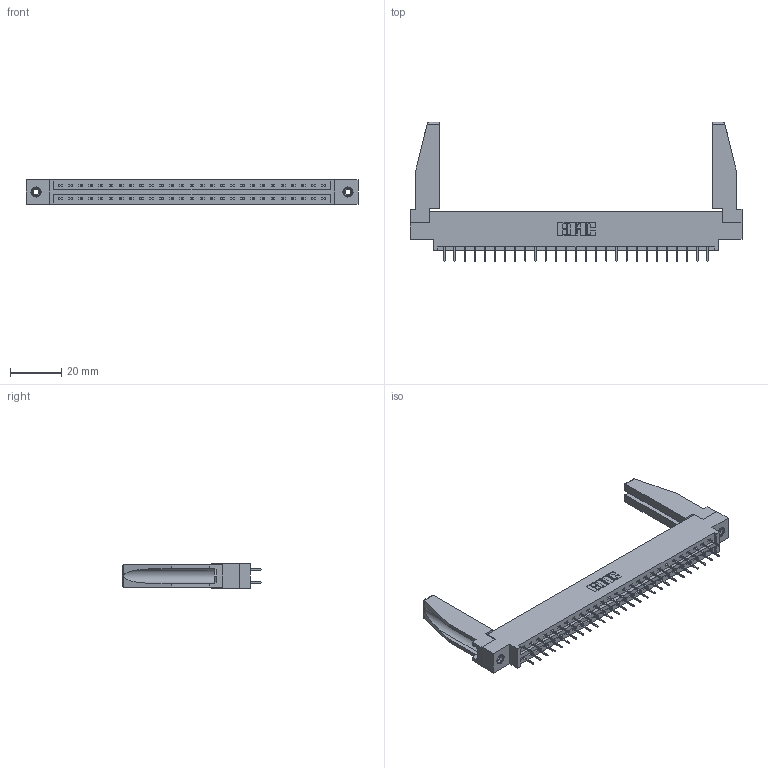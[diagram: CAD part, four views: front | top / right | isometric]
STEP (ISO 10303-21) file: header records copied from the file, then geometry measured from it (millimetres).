
FILE_DESCRIPTION (( 'STEP AP203' ), '1' );
FILE_NAME ('387-054-524-878.STEP', '2019-10-19T04:49:30', ( '' ), ( '' ), 'SwSTEP 2.0', 'SolidWorks 2016', '' );
FILE_SCHEMA (( 'CONFIG_CONTROL_DESIGN' ));
Length unit declared in the file: inch
Products named in the file (5): 307-220-078; 345-292-001_345-293-124; 337 Part_0.170 Offset - 0.156 Dia-TI; 387-054-524-878; 345-250-001_345-250-001-102
Assembly tree (59 placements, depth 2):
  387-054-524-878
    337 Part_0.170 Offset - 0.156 Dia-TI
    345-292-001_345-293-124  x54
    345-250-001_345-250-001-102  x2
    307-220-078  x2
Bounding box: 130 x 54.49 x 9.4 mm (x, y, z)
Volume: 17294.6 mm3; surface area: 18576.6 mm2
Topology: 59 solids, 59 shells, 3380 faces, 9563 edges, 6150 vertices
Faces by surface type: plane 2534, cylinder 830, cone 12, torus 4
Entity records: 25520 total; most frequent: CARTESIAN_POINT 4312, ORIENTED_EDGE 4204, DIRECTION 3702, EDGE_CURVE 2102, LINE 1940, VECTOR 1940, VERTEX_POINT 1392, AXIS2_PLACEMENT_3D 881
